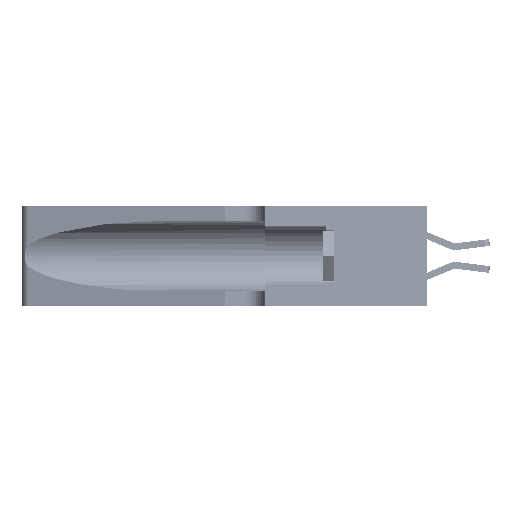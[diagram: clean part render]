
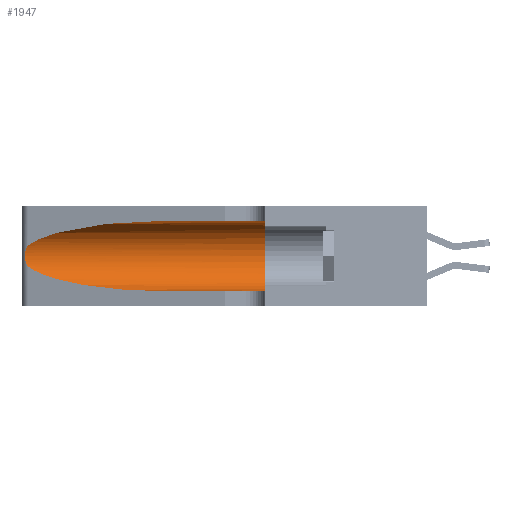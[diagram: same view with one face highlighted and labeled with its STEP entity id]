
A CAD part, left-side view. The second image highlights one B-rep face of the part: STEP entity #1947.
In plain terms, the highlighted cylindrical face has radius 3.308 mm (diameter 6.617 mm), a partial arc.
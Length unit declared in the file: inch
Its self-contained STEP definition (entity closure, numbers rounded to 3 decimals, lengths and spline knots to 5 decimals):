
#512 = EDGE_CURVE ( 'NONE', #42714, #43716, #35311, .T. ) ;
#1581 = EDGE_CURVE ( 'NONE', #42714, #18641, #4744, .T. ) ;
#1932 = CARTESIAN_POINT ( 'NONE',  ( 0.25555, 1.22994, 0.2215 ) ) ;
#1947 = ADVANCED_FACE ( 'NONE', ( #47537 ), #36443, .F. ) ;
#2105 = CARTESIAN_POINT ( 'NONE',  ( 0.25555, 1.22993, 0.14849 ) ) ;
#2168 = ORIENTED_EDGE ( 'NONE', *, *, #38005, .F. ) ;
#2399 = VECTOR ( 'NONE', #25000, 39.37008 ) ;
#2836 = CARTESIAN_POINT ( 'NONE',  ( 0.2373, 1.15595, 0.08982 ) ) ;
#4744 = LINE ( 'NONE', #43556, #2399 ) ;
#8630 = VECTOR ( 'NONE', #32821, 39.37008 ) ;
#8666 = CARTESIAN_POINT ( 'NONE',  ( 0.1305, 0.35, 0.31525 ) ) ;
#9526 = CARTESIAN_POINT ( 'NONE',  ( 0.25787, 1.23484, 0.2124 ) ) ;
#12296 = DIRECTION ( 'NONE',  ( 0., 1., 0. ) ) ;
#12601 = AXIS2_PLACEMENT_3D ( 'NONE', #15614, #23201, #41735 ) ;
#13324 = EDGE_CURVE ( 'NONE', #45578, #23485, #48406, .T. ) ;
#13347 = CARTESIAN_POINT ( 'NONE',  ( 0.26018, 1.23835, 0.19895 ) ) ;
#14232 = CARTESIAN_POINT ( 'NONE',  ( 0.25487, 1.22718, 0.14631 ) ) ;
#15614 = CARTESIAN_POINT ( 'NONE',  ( 0.1305, 1.61858, 0.185 ) ) ;
#17112 = CARTESIAN_POINT ( 'NONE',  ( 0.26075, 1.23896, 0.178 ) ) ;
#17286 = CARTESIAN_POINT ( 'NONE',  ( 0.2373, 1.15595, 0.28018 ) ) ;
#17593 = EDGE_CURVE ( 'NONE', #24199, #45578, #38408, .T. ) ;
#18641 = VERTEX_POINT ( 'NONE', #8666 ) ;
#20026 = CARTESIAN_POINT ( 'NONE',  ( 0.25487, 1.22718, 0.22369 ) ) ;
#20906 = CARTESIAN_POINT ( 'NONE',  ( 0.25856, 1.23593, 0.16098 ) ) ;
#21079 = CARTESIAN_POINT ( 'NONE',  ( 0.25487, 1.22718, 0.22369 ) ) ;
#22250 = ORIENTED_EDGE ( 'NONE', *, *, #17593, .T. ) ;
#22572 = B_SPLINE_CURVE_WITH_KNOTS ( 'NONE', 3,
 ( #46786, #1932, #31969, #9526, #35698, #13347, #39458, #17112, #43194, #20906, #46954, #24652, #2105, #28388 ),
 .UNSPECIFIED., .F., .F.,
 ( 4, 2, 2, 2, 2, 2, 4 ),
 ( 0., 0.00027, 0.00053, 0.00107, 0.0016, 0.00187, 0.00214 ),
 .UNSPECIFIED. ) ;
#23201 = DIRECTION ( 'NONE',  ( 0., -1., 0. ) ) ;
#23485 = VERTEX_POINT ( 'NONE', #25891 ) ;
#24199 = VERTEX_POINT ( 'NONE', #37066 ) ;
#24652 = CARTESIAN_POINT ( 'NONE',  ( 0.25639, 1.23186, 0.15144 ) ) ;
#25000 = DIRECTION ( 'NONE',  ( 0., -1., 0. ) ) ;
#25716 = ORIENTED_EDGE ( 'NONE', *, *, #37414, .T. ) ;
#25891 = CARTESIAN_POINT ( 'NONE',  ( 0.1305, 0.35, 0.05475 ) ) ;
#28254 = CIRCLE ( 'NONE', #40352, 0.13025 ) ;
#28388 = CARTESIAN_POINT ( 'NONE',  ( 0.25487, 1.22718, 0.14631 ) ) ;
#29485 = EDGE_LOOP ( 'NONE', ( #45521, #25716, #22250, #41419, #2168, #41228 ) ) ;
#31969 = CARTESIAN_POINT ( 'NONE',  ( 0.25639, 1.23184, 0.21858 ) ) ;
#32821 = DIRECTION ( 'NONE',  ( 0., -1., 0. ) ) ;
#32842 = CARTESIAN_POINT ( 'NONE',  ( 0.18966, 0.96281, 0.05475 ) ) ;
#34666 = CARTESIAN_POINT ( 'NONE',  ( 0.1305, 0.35, 0.185 ) ) ;
#35311 =( BOUNDED_CURVE ( )  B_SPLINE_CURVE ( 3, ( #43356, #39620, #17286, #21079 ),
 .UNSPECIFIED., .F., .T. ) 
 B_SPLINE_CURVE_WITH_KNOTS ( ( 4, 4 ),
 ( 1.5708, 2.84003 ),
 .UNSPECIFIED. ) 
 CURVE ( )  GEOMETRIC_REPRESENTATION_ITEM ( )  RATIONAL_B_SPLINE_CURVE ( ( 1., 0.87, 0.87, 1. ) ) 
 REPRESENTATION_ITEM ( '' )  );
#35698 = CARTESIAN_POINT ( 'NONE',  ( 0.25854, 1.2359, 0.20912 ) ) ;
#36443 = CYLINDRICAL_SURFACE ( 'NONE', #12601, 0.13025 ) ;
#37066 = CARTESIAN_POINT ( 'NONE',  ( 0.25487, 1.22718, 0.14631 ) ) ;
#37414 = EDGE_CURVE ( 'NONE', #43716, #24199, #22572, .T. ) ;
#38005 = EDGE_CURVE ( 'NONE', #18641, #23485, #28254, .T. ) ;
#38408 =( BOUNDED_CURVE ( )  B_SPLINE_CURVE ( 3, ( #14232, #2836, #32842, #40337 ),
 .UNSPECIFIED., .F., .T. ) 
 B_SPLINE_CURVE_WITH_KNOTS ( ( 4, 4 ),
 ( 3.44316, 4.71239 ),
 .UNSPECIFIED. ) 
 CURVE ( )  GEOMETRIC_REPRESENTATION_ITEM ( )  RATIONAL_B_SPLINE_CURVE ( ( 1., 0.87, 0.87, 1. ) ) 
 REPRESENTATION_ITEM ( '' )  );
#38424 = DIRECTION ( 'NONE',  ( 0., 0., 1. ) ) ;
#39458 = CARTESIAN_POINT ( 'NONE',  ( 0.26075, 1.23896, 0.19203 ) ) ;
#39620 = CARTESIAN_POINT ( 'NONE',  ( 0.18966, 0.96281, 0.31525 ) ) ;
#40156 = CARTESIAN_POINT ( 'NONE',  ( 0.1305, 1.61858, 0.05475 ) ) ;
#40337 = CARTESIAN_POINT ( 'NONE',  ( 0.1305, 0.72297, 0.05475 ) ) ;
#40352 = AXIS2_PLACEMENT_3D ( 'NONE', #34666, #12296, #38424 ) ;
#41228 = ORIENTED_EDGE ( 'NONE', *, *, #1581, .F. ) ;
#41419 = ORIENTED_EDGE ( 'NONE', *, *, #13324, .T. ) ;
#41633 = CARTESIAN_POINT ( 'NONE',  ( 0.1305, 0.72297, 0.05475 ) ) ;
#41735 = DIRECTION ( 'NONE',  ( 0., 0., -1. ) ) ;
#42714 = VERTEX_POINT ( 'NONE', #44063 ) ;
#43194 = CARTESIAN_POINT ( 'NONE',  ( 0.26017, 1.23833, 0.17102 ) ) ;
#43356 = CARTESIAN_POINT ( 'NONE',  ( 0.1305, 0.72297, 0.31525 ) ) ;
#43556 = CARTESIAN_POINT ( 'NONE',  ( 0.1305, 1.61858, 0.31525 ) ) ;
#43716 = VERTEX_POINT ( 'NONE', #20026 ) ;
#44063 = CARTESIAN_POINT ( 'NONE',  ( 0.1305, 0.72297, 0.31525 ) ) ;
#45521 = ORIENTED_EDGE ( 'NONE', *, *, #512, .T. ) ;
#45578 = VERTEX_POINT ( 'NONE', #41633 ) ;
#46786 = CARTESIAN_POINT ( 'NONE',  ( 0.25487, 1.22718, 0.22369 ) ) ;
#46954 = CARTESIAN_POINT ( 'NONE',  ( 0.25789, 1.23486, 0.15765 ) ) ;
#47537 = FACE_OUTER_BOUND ( 'NONE', #29485, .T. ) ;
#48406 = LINE ( 'NONE', #40156, #8630 ) ;
